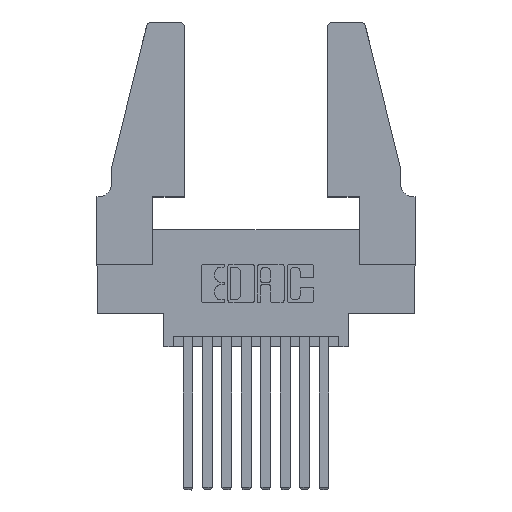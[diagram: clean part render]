
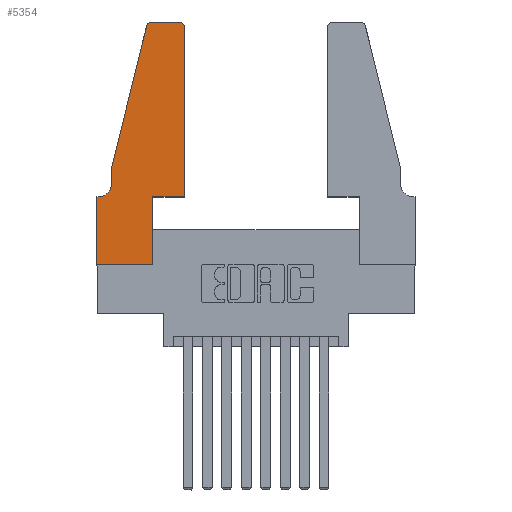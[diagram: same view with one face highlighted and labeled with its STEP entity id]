
A CAD part, top view. The second image highlights one B-rep face of the part: STEP entity #5354.
In plain terms, the highlighted planar face has unit normal (0, 0, 1).
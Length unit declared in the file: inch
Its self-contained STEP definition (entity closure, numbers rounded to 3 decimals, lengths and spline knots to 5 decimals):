
#278 = CARTESIAN_POINT ( 'NONE',  ( 0.2865, 0., 0.37 ) ) ;
#319 = EDGE_CURVE ( 'NONE', #4657, #6425, #5955, .T. ) ;
#485 = ORIENTED_EDGE ( 'NONE', *, *, #3853, .T. ) ;
#816 = VERTEX_POINT ( 'NONE', #877 ) ;
#877 = CARTESIAN_POINT ( 'NONE',  ( 0., 0.35, 0.37 ) ) ;
#882 = ORIENTED_EDGE ( 'NONE', *, *, #7405, .T. ) ;
#888 = DIRECTION ( 'NONE',  ( 1., 0., 0. ) ) ;
#919 = VERTEX_POINT ( 'NONE', #6242 ) ;
#1001 = CIRCLE ( 'NONE', #9153, 0.03 ) ;
#1087 = CARTESIAN_POINT ( 'NONE',  ( 0.0755, 0.42, 0.37 ) ) ;
#1234 = LINE ( 'NONE', #2441, #1681 ) ;
#1243 = ORIENTED_EDGE ( 'NONE', *, *, #319, .T. ) ;
#1250 = AXIS2_PLACEMENT_3D ( 'NONE', #12464, #3458, #1387 ) ;
#1387 = DIRECTION ( 'NONE',  ( 1., 0., 0. ) ) ;
#1432 = CARTESIAN_POINT ( 'NONE',  ( 0.4505, 0.35, 0.37 ) ) ;
#1573 = CARTESIAN_POINT ( 'NONE',  ( 0.4505, 0.35, 0.37 ) ) ;
#1681 = VECTOR ( 'NONE', #11464, 39.37008 ) ;
#1803 = DIRECTION ( 'NONE',  ( -0.239, -0.971, 0. ) ) ;
#1814 = ORIENTED_EDGE ( 'NONE', *, *, #6487, .T. ) ;
#1878 = DIRECTION ( 'NONE',  ( 0., -1., 0. ) ) ;
#1945 = ORIENTED_EDGE ( 'NONE', *, *, #11192, .T. ) ;
#2441 = CARTESIAN_POINT ( 'NONE',  ( 0., 0., 0.37 ) ) ;
#2777 = CARTESIAN_POINT ( 'NONE',  ( 0., 0., 0.37 ) ) ;
#3458 = DIRECTION ( 'NONE',  ( 0., 0., 1. ) ) ;
#3499 = CARTESIAN_POINT ( 'NONE',  ( 0.0755, 0.35, 0.37 ) ) ;
#3614 = CARTESIAN_POINT ( 'NONE',  ( 0.4505, 1.22, 0.37 ) ) ;
#3676 = LINE ( 'NONE', #3499, #5704 ) ;
#3686 = ORIENTED_EDGE ( 'NONE', *, *, #6756, .T. ) ;
#3698 = EDGE_CURVE ( 'NONE', #7189, #5342, #9189, .T. ) ;
#3838 = VECTOR ( 'NONE', #9413, 39.37008 ) ;
#3853 = EDGE_CURVE ( 'NONE', #12927, #816, #3676, .T. ) ;
#4074 = VECTOR ( 'NONE', #8604, 39.37008 ) ;
#4309 = VERTEX_POINT ( 'NONE', #10722 ) ;
#4341 = LINE ( 'NONE', #2777, #9668 ) ;
#4473 = ORIENTED_EDGE ( 'NONE', *, *, #4901, .T. ) ;
#4657 = VERTEX_POINT ( 'NONE', #11297 ) ;
#4861 = DIRECTION ( 'NONE',  ( 0., 0., 1. ) ) ;
#4901 = EDGE_CURVE ( 'NONE', #8067, #6199, #1001, .T. ) ;
#5127 = CIRCLE ( 'NONE', #11333, 0.03 ) ;
#5342 = VERTEX_POINT ( 'NONE', #1432 ) ;
#5354 = ADVANCED_FACE ( 'NONE', ( #12730 ), #6416, .T. ) ;
#5486 = LINE ( 'NONE', #5980, #8636 ) ;
#5499 = VERTEX_POINT ( 'NONE', #278 ) ;
#5704 = VECTOR ( 'NONE', #12498, 39.37008 ) ;
#5725 = CARTESIAN_POINT ( 'NONE',  ( 0.4205, 1.22, 0.37 ) ) ;
#5814 = ORIENTED_EDGE ( 'NONE', *, *, #12793, .T. ) ;
#5882 = CARTESIAN_POINT ( 'NONE',  ( 0.0755, 0.5, 0.37 ) ) ;
#5955 = LINE ( 'NONE', #9266, #9600 ) ;
#5980 = CARTESIAN_POINT ( 'NONE',  ( 0.2865, 0.35, 0.37 ) ) ;
#6199 = VERTEX_POINT ( 'NONE', #12650 ) ;
#6242 = CARTESIAN_POINT ( 'NONE',  ( 0., 0., 0.37 ) ) ;
#6357 = EDGE_CURVE ( 'NONE', #6199, #10814, #7847, .T. ) ;
#6416 = PLANE ( 'NONE',  #1250 ) ;
#6425 = VERTEX_POINT ( 'NONE', #1087 ) ;
#6487 = EDGE_CURVE ( 'NONE', #6425, #12927, #7549, .T. ) ;
#6743 = VECTOR ( 'NONE', #1803, 39.37008 ) ;
#6756 = EDGE_CURVE ( 'NONE', #5499, #7189, #5486, .T. ) ;
#7189 = VERTEX_POINT ( 'NONE', #8031 ) ;
#7305 = CARTESIAN_POINT ( 'NONE',  ( 0.4505, 0.35, 0.37 ) ) ;
#7360 = DIRECTION ( 'NONE',  ( 0., 1., 0. ) ) ;
#7405 = EDGE_CURVE ( 'NONE', #5342, #8067, #11426, .T. ) ;
#7549 = CIRCLE ( 'NONE', #8809, 0.07 ) ;
#7709 = CARTESIAN_POINT ( 'NONE',  ( 0.284, 1.22, 0.37 ) ) ;
#7740 = DIRECTION ( 'NONE',  ( 0., 0., 1. ) ) ;
#7847 = LINE ( 'NONE', #9204, #9285 ) ;
#8031 = CARTESIAN_POINT ( 'NONE',  ( 0.2865, 0.35, 0.37 ) ) ;
#8067 = VERTEX_POINT ( 'NONE', #3614 ) ;
#8332 = DIRECTION ( 'NONE',  ( 0., 0., -1. ) ) ;
#8394 = EDGE_CURVE ( 'NONE', #10814, #4309, #5127, .T. ) ;
#8426 = CARTESIAN_POINT ( 'NONE',  ( 0.0055, 0.42, 0.37 ) ) ;
#8604 = DIRECTION ( 'NONE',  ( 0., 1., 0. ) ) ;
#8636 = VECTOR ( 'NONE', #7360, 39.37008 ) ;
#8809 = AXIS2_PLACEMENT_3D ( 'NONE', #8426, #8332, #9453 ) ;
#8879 = CARTESIAN_POINT ( 'NONE',  ( 0.284, 1.25, 0.37 ) ) ;
#9153 = AXIS2_PLACEMENT_3D ( 'NONE', #5725, #7740, #9813 ) ;
#9155 = DIRECTION ( 'NONE',  ( -1., 0., 0. ) ) ;
#9189 = LINE ( 'NONE', #7305, #3838 ) ;
#9204 = CARTESIAN_POINT ( 'NONE',  ( 0.2605, 1.25, 0.37 ) ) ;
#9265 = EDGE_CURVE ( 'NONE', #816, #919, #4341, .T. ) ;
#9266 = CARTESIAN_POINT ( 'NONE',  ( 0.0755, 0.5, 0.37 ) ) ;
#9285 = VECTOR ( 'NONE', #9155, 39.37008 ) ;
#9413 = DIRECTION ( 'NONE',  ( 1., 0., 0. ) ) ;
#9453 = DIRECTION ( 'NONE',  ( -1., 0., 0. ) ) ;
#9600 = VECTOR ( 'NONE', #12260, 39.37008 ) ;
#9668 = VECTOR ( 'NONE', #1878, 39.37008 ) ;
#9813 = DIRECTION ( 'NONE',  ( 1., 0., 0. ) ) ;
#10049 = EDGE_LOOP ( 'NONE', ( #11160, #10403, #1945, #1243, #1814, #485, #12614, #5814, #3686, #11314, #882, #4473 ) ) ;
#10403 = ORIENTED_EDGE ( 'NONE', *, *, #8394, .T. ) ;
#10722 = CARTESIAN_POINT ( 'NONE',  ( 0.25487, 1.22718, 0.37 ) ) ;
#10814 = VERTEX_POINT ( 'NONE', #8879 ) ;
#11160 = ORIENTED_EDGE ( 'NONE', *, *, #6357, .T. ) ;
#11192 = EDGE_CURVE ( 'NONE', #4309, #4657, #12842, .T. ) ;
#11297 = CARTESIAN_POINT ( 'NONE',  ( 0.0755, 0.5, 0.37 ) ) ;
#11314 = ORIENTED_EDGE ( 'NONE', *, *, #3698, .T. ) ;
#11333 = AXIS2_PLACEMENT_3D ( 'NONE', #7709, #4861, #888 ) ;
#11426 = LINE ( 'NONE', #1573, #4074 ) ;
#11464 = DIRECTION ( 'NONE',  ( 1., 0., 0. ) ) ;
#12260 = DIRECTION ( 'NONE',  ( 0., -1., 0. ) ) ;
#12464 = CARTESIAN_POINT ( 'NONE',  ( 0., 0.35, 0.37 ) ) ;
#12498 = DIRECTION ( 'NONE',  ( -1., 0., 0. ) ) ;
#12614 = ORIENTED_EDGE ( 'NONE', *, *, #9265, .T. ) ;
#12650 = CARTESIAN_POINT ( 'NONE',  ( 0.4205, 1.25, 0.37 ) ) ;
#12670 = CARTESIAN_POINT ( 'NONE',  ( 0.0055, 0.35, 0.37 ) ) ;
#12730 = FACE_OUTER_BOUND ( 'NONE', #10049, .T. ) ;
#12793 = EDGE_CURVE ( 'NONE', #919, #5499, #1234, .T. ) ;
#12842 = LINE ( 'NONE', #5882, #6743 ) ;
#12927 = VERTEX_POINT ( 'NONE', #12670 ) ;
